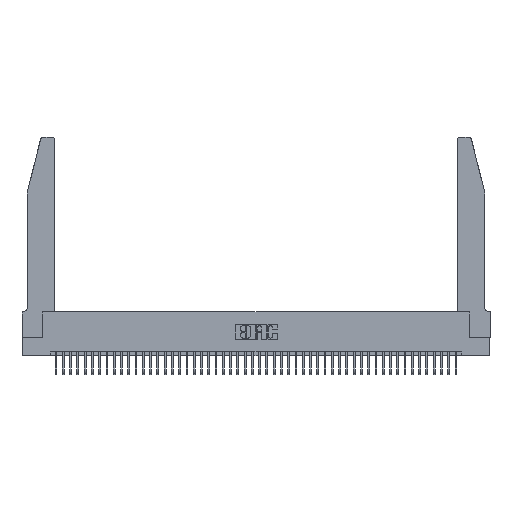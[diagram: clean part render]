
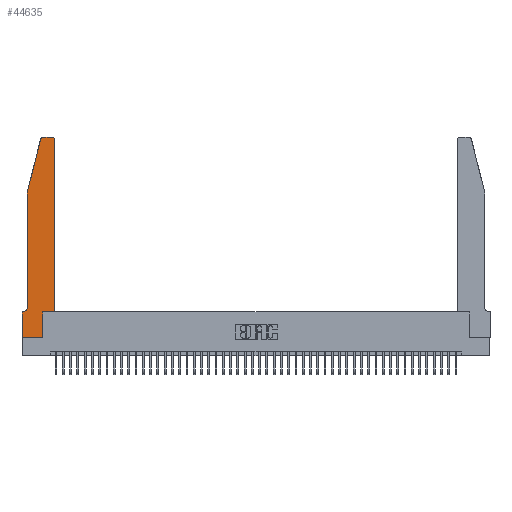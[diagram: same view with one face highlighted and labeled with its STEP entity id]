
A CAD part, top view. The second image highlights one B-rep face of the part: STEP entity #44635.
In plain terms, the highlighted planar face has unit normal (0, 0, 1).
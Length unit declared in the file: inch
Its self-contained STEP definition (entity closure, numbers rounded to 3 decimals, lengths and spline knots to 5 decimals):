
#494 = DIRECTION ( 'NONE',  ( 0., 0., 1. ) ) ;
#696 = EDGE_CURVE ( 'NONE', #21530, #30661, #9461, .T. ) ;
#785 = DIRECTION ( 'NONE',  ( 0., 1., 0. ) ) ;
#2405 = AXIS2_PLACEMENT_3D ( 'NONE', #21491, #494, #24967 ) ;
#2570 = VERTEX_POINT ( 'NONE', #27005 ) ;
#2931 = ORIENTED_EDGE ( 'NONE', *, *, #32592, .T. ) ;
#2985 = VECTOR ( 'NONE', #7762, 39.37008 ) ;
#4102 = CIRCLE ( 'NONE', #17641, 0.07 ) ;
#4219 = CARTESIAN_POINT ( 'NONE',  ( 0.4505, 0.35, 0.37 ) ) ;
#4344 = AXIS2_PLACEMENT_3D ( 'NONE', #17716, #41896, #21201 ) ;
#6128 = VECTOR ( 'NONE', #785, 39.37008 ) ;
#6842 = CARTESIAN_POINT ( 'NONE',  ( 0., 0.35, 0.37 ) ) ;
#7192 = LINE ( 'NONE', #34861, #33859 ) ;
#7405 = CARTESIAN_POINT ( 'NONE',  ( 0.0755, 0.35, 0.37 ) ) ;
#7448 = PLANE ( 'NONE',  #2405 ) ;
#7493 = LINE ( 'NONE', #12452, #16795 ) ;
#7699 = VERTEX_POINT ( 'NONE', #37223 ) ;
#7762 = DIRECTION ( 'NONE',  ( 1., 0., 0. ) ) ;
#7925 = EDGE_CURVE ( 'NONE', #7699, #13357, #22971, .T. ) ;
#8401 = DIRECTION ( 'NONE',  ( 0., -1., 0. ) ) ;
#8843 = CARTESIAN_POINT ( 'NONE',  ( 0.4505, 0.35, 0.37 ) ) ;
#9461 = LINE ( 'NONE', #7405, #17667 ) ;
#10766 = DIRECTION ( 'NONE',  ( -0.239, -0.971, 0. ) ) ;
#11151 = ORIENTED_EDGE ( 'NONE', *, *, #27989, .T. ) ;
#11372 = DIRECTION ( 'NONE',  ( -1., 0., 0. ) ) ;
#11402 = CARTESIAN_POINT ( 'NONE',  ( 0.284, 2.75, 0.37 ) ) ;
#12283 = ORIENTED_EDGE ( 'NONE', *, *, #14712, .T. ) ;
#12452 = CARTESIAN_POINT ( 'NONE',  ( 0., 0., 0.37 ) ) ;
#12663 = ORIENTED_EDGE ( 'NONE', *, *, #31882, .T. ) ;
#13342 = VERTEX_POINT ( 'NONE', #24893 ) ;
#13357 = VERTEX_POINT ( 'NONE', #42120 ) ;
#13892 = VERTEX_POINT ( 'NONE', #14225 ) ;
#14225 = CARTESIAN_POINT ( 'NONE',  ( 0.4505, 0.35, 0.37 ) ) ;
#14230 = AXIS2_PLACEMENT_3D ( 'NONE', #18937, #43119, #22415 ) ;
#14712 = EDGE_CURVE ( 'NONE', #39795, #21530, #4102, .T. ) ;
#14726 = VECTOR ( 'NONE', #19408, 39.37008 ) ;
#14942 = CARTESIAN_POINT ( 'NONE',  ( 0.0755, 0.42, 0.37 ) ) ;
#15094 = ORIENTED_EDGE ( 'NONE', *, *, #18290, .T. ) ;
#15413 = VECTOR ( 'NONE', #28326, 39.37008 ) ;
#15418 = LINE ( 'NONE', #21772, #6128 ) ;
#15832 = CARTESIAN_POINT ( 'NONE',  ( 0.0055, 0.42, 0.37 ) ) ;
#16795 = VECTOR ( 'NONE', #29751, 39.37008 ) ;
#17641 = AXIS2_PLACEMENT_3D ( 'NONE', #15832, #40062, #19370 ) ;
#17667 = VECTOR ( 'NONE', #17815, 39.37008 ) ;
#17716 = CARTESIAN_POINT ( 'NONE',  ( 0.4205, 2.72, 0.37 ) ) ;
#17815 = DIRECTION ( 'NONE',  ( -1., 0., 0. ) ) ;
#18290 = EDGE_CURVE ( 'NONE', #43721, #13342, #44535, .T. ) ;
#18937 = CARTESIAN_POINT ( 'NONE',  ( 0.284, 2.72, 0.37 ) ) ;
#18986 = VECTOR ( 'NONE', #11372, 39.37008 ) ;
#19237 = ORIENTED_EDGE ( 'NONE', *, *, #696, .T. ) ;
#19370 = DIRECTION ( 'NONE',  ( -1., 0., 0. ) ) ;
#19408 = DIRECTION ( 'NONE',  ( 0., 1., 0. ) ) ;
#19509 = EDGE_CURVE ( 'NONE', #13892, #7699, #42364, .T. ) ;
#21201 = DIRECTION ( 'NONE',  ( 1., 0., 0. ) ) ;
#21284 = EDGE_CURVE ( 'NONE', #40742, #13892, #21615, .T. ) ;
#21491 = CARTESIAN_POINT ( 'NONE',  ( 0., 0.35, 0.37 ) ) ;
#21530 = VERTEX_POINT ( 'NONE', #29968 ) ;
#21615 = LINE ( 'NONE', #4219, #2985 ) ;
#21772 = CARTESIAN_POINT ( 'NONE',  ( 0.2865, 0.35, 0.37 ) ) ;
#22415 = DIRECTION ( 'NONE',  ( 1., 0., 0. ) ) ;
#22971 = CIRCLE ( 'NONE', #4344, 0.03 ) ;
#24131 = ORIENTED_EDGE ( 'NONE', *, *, #24525, .T. ) ;
#24296 = EDGE_LOOP ( 'NONE', ( #11151, #15094, #12663, #42134, #12283, #19237, #2931, #43067, #24131, #26445, #40525, #36177 ) ) ;
#24525 = EDGE_CURVE ( 'NONE', #2570, #40742, #15418, .T. ) ;
#24893 = CARTESIAN_POINT ( 'NONE',  ( 0.25487, 2.72718, 0.37 ) ) ;
#24965 = CARTESIAN_POINT ( 'NONE',  ( 0., 0., 0.37 ) ) ;
#24967 = DIRECTION ( 'NONE',  ( 1., 0., 0. ) ) ;
#25190 = CARTESIAN_POINT ( 'NONE',  ( 0.2605, 2.75, 0.37 ) ) ;
#26445 = ORIENTED_EDGE ( 'NONE', *, *, #21284, .T. ) ;
#27005 = CARTESIAN_POINT ( 'NONE',  ( 0.2865, 0., 0.37 ) ) ;
#27989 = EDGE_CURVE ( 'NONE', #13357, #43721, #35207, .T. ) ;
#28326 = DIRECTION ( 'NONE',  ( 0., -1., 0. ) ) ;
#29155 = VERTEX_POINT ( 'NONE', #34469 ) ;
#29751 = DIRECTION ( 'NONE',  ( 1., 0., 0. ) ) ;
#29968 = CARTESIAN_POINT ( 'NONE',  ( 0.0055, 0.35, 0.37 ) ) ;
#30661 = VERTEX_POINT ( 'NONE', #6842 ) ;
#31882 = EDGE_CURVE ( 'NONE', #13342, #37406, #7192, .T. ) ;
#32067 = EDGE_CURVE ( 'NONE', #37406, #39795, #44603, .T. ) ;
#32592 = EDGE_CURVE ( 'NONE', #30661, #29155, #33865, .T. ) ;
#33631 = CARTESIAN_POINT ( 'NONE',  ( 0.0755, 2., 0.37 ) ) ;
#33859 = VECTOR ( 'NONE', #10766, 39.37008 ) ;
#33865 = LINE ( 'NONE', #24965, #15413 ) ;
#34469 = CARTESIAN_POINT ( 'NONE',  ( 0., 0., 0.37 ) ) ;
#34861 = CARTESIAN_POINT ( 'NONE',  ( 0.0755, 2., 0.37 ) ) ;
#35207 = LINE ( 'NONE', #25190, #18986 ) ;
#35441 = VECTOR ( 'NONE', #8401, 39.37008 ) ;
#36177 = ORIENTED_EDGE ( 'NONE', *, *, #7925, .T. ) ;
#37223 = CARTESIAN_POINT ( 'NONE',  ( 0.4505, 2.72, 0.37 ) ) ;
#37406 = VERTEX_POINT ( 'NONE', #33631 ) ;
#39524 = CARTESIAN_POINT ( 'NONE',  ( 0.0755, 2., 0.37 ) ) ;
#39795 = VERTEX_POINT ( 'NONE', #14942 ) ;
#40062 = DIRECTION ( 'NONE',  ( 0., 0., -1. ) ) ;
#40503 = EDGE_CURVE ( 'NONE', #29155, #2570, #7493, .T. ) ;
#40525 = ORIENTED_EDGE ( 'NONE', *, *, #19509, .T. ) ;
#40742 = VERTEX_POINT ( 'NONE', #42409 ) ;
#41896 = DIRECTION ( 'NONE',  ( 0., 0., 1. ) ) ;
#42120 = CARTESIAN_POINT ( 'NONE',  ( 0.4205, 2.75, 0.37 ) ) ;
#42134 = ORIENTED_EDGE ( 'NONE', *, *, #32067, .T. ) ;
#42364 = LINE ( 'NONE', #8843, #14726 ) ;
#42409 = CARTESIAN_POINT ( 'NONE',  ( 0.2865, 0.35, 0.37 ) ) ;
#43067 = ORIENTED_EDGE ( 'NONE', *, *, #40503, .T. ) ;
#43119 = DIRECTION ( 'NONE',  ( 0., 0., 1. ) ) ;
#43721 = VERTEX_POINT ( 'NONE', #11402 ) ;
#44206 = FACE_OUTER_BOUND ( 'NONE', #24296, .T. ) ;
#44535 = CIRCLE ( 'NONE', #14230, 0.03 ) ;
#44603 = LINE ( 'NONE', #39524, #35441 ) ;
#44635 = ADVANCED_FACE ( 'NONE', ( #44206 ), #7448, .T. ) ;
